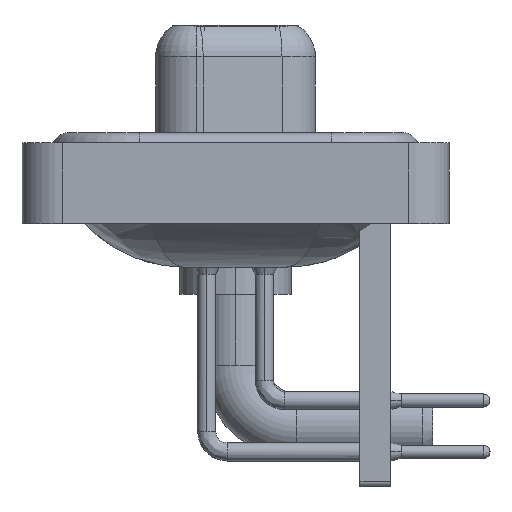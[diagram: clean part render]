
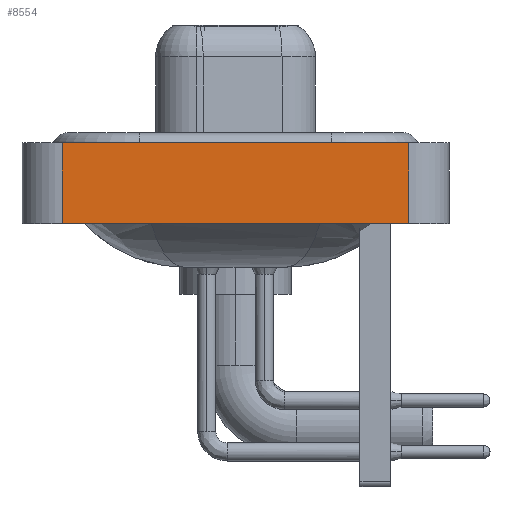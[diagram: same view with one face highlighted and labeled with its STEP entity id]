
A CAD part, left-side view. The second image highlights one B-rep face of the part: STEP entity #8554.
In plain terms, the highlighted planar face has unit normal (-1, 0, 0).
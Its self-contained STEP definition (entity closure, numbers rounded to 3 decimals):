
#315 = VERTEX_POINT ( 'NONE', #11650 ) ;
#452 = EDGE_LOOP ( 'NONE', ( #15605, #2983, #18445, #2498 ) ) ;
#1960 = VERTEX_POINT ( 'NONE', #10857 ) ;
#2055 = VERTEX_POINT ( 'NONE', #20121 ) ;
#2498 = ORIENTED_EDGE ( 'NONE', *, *, #23205, .T. ) ;
#2983 = ORIENTED_EDGE ( 'NONE', *, *, #22000, .F. ) ;
#5030 = CARTESIAN_POINT ( 'NONE',  ( -7.35, -8.55, -3.6 ) ) ;
#5288 = DIRECTION ( 'NONE',  ( 0., 0., 1. ) ) ;
#5502 = DIRECTION ( 'NONE',  ( 0., 0., 1. ) ) ;
#5979 = PLANE ( 'NONE',  #13561 ) ;
#7842 = LINE ( 'NONE', #24467, #20696 ) ;
#8554 = ADVANCED_FACE ( 'NONE', ( #21022 ), #5979, .T. ) ;
#8592 = DIRECTION ( 'NONE',  ( -1., 0., 0. ) ) ;
#8877 = LINE ( 'NONE', #5030, #25414 ) ;
#10857 = CARTESIAN_POINT ( 'NONE',  ( -7.35, -8.55, 0.4 ) ) ;
#11527 = LINE ( 'NONE', #26712, #11569 ) ;
#11569 = VECTOR ( 'NONE', #26189, 1000. ) ;
#11650 = CARTESIAN_POINT ( 'NONE',  ( -7.35, 8.55, 0.4 ) ) ;
#13561 = AXIS2_PLACEMENT_3D ( 'NONE', #14376, #8592, #16480 ) ;
#13598 = LINE ( 'NONE', #22061, #24328 ) ;
#14376 = CARTESIAN_POINT ( 'NONE',  ( -7.35, -8.55, -3.6 ) ) ;
#15442 = CARTESIAN_POINT ( 'NONE',  ( -7.35, -8.55, -3.6 ) ) ;
#15605 = ORIENTED_EDGE ( 'NONE', *, *, #15892, .T. ) ;
#15892 = EDGE_CURVE ( 'NONE', #17176, #1960, #8877, .T. ) ;
#16480 = DIRECTION ( 'NONE',  ( 0., 0., 1. ) ) ;
#17176 = VERTEX_POINT ( 'NONE', #15442 ) ;
#17441 = EDGE_CURVE ( 'NONE', #2055, #315, #7842, .T. ) ;
#18445 = ORIENTED_EDGE ( 'NONE', *, *, #17441, .F. ) ;
#20121 = CARTESIAN_POINT ( 'NONE',  ( -7.35, 8.55, -3.6 ) ) ;
#20696 = VECTOR ( 'NONE', #5502, 1000. ) ;
#21022 = FACE_OUTER_BOUND ( 'NONE', #452, .T. ) ;
#22000 = EDGE_CURVE ( 'NONE', #315, #1960, #11527, .T. ) ;
#22061 = CARTESIAN_POINT ( 'NONE',  ( -7.35, -8.55, -3.6 ) ) ;
#23205 = EDGE_CURVE ( 'NONE', #2055, #17176, #13598, .T. ) ;
#24328 = VECTOR ( 'NONE', #24785, 1000. ) ;
#24467 = CARTESIAN_POINT ( 'NONE',  ( -7.35, 8.55, -3.6 ) ) ;
#24785 = DIRECTION ( 'NONE',  ( 0., -1., 0. ) ) ;
#25414 = VECTOR ( 'NONE', #5288, 1000. ) ;
#26189 = DIRECTION ( 'NONE',  ( 0., -1., 0. ) ) ;
#26712 = CARTESIAN_POINT ( 'NONE',  ( -7.35, -8.55, 0.4 ) ) ;
